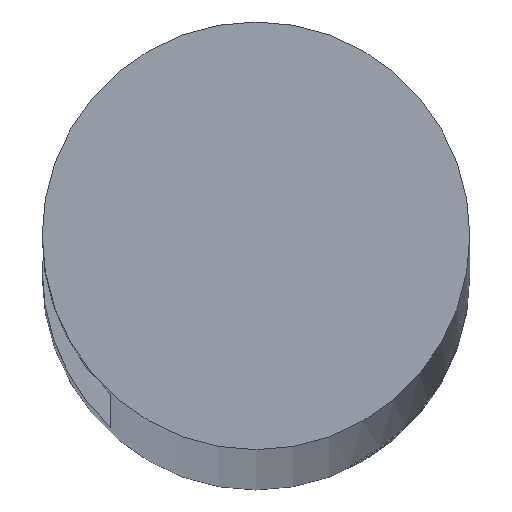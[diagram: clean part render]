
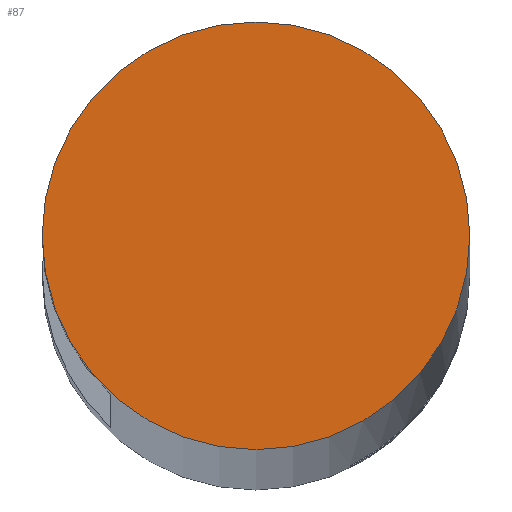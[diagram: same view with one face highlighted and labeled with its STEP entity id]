
A CAD part, top view. The second image highlights one B-rep face of the part: STEP entity #87.
In plain terms, the highlighted planar face has unit normal (0, 0, 1).
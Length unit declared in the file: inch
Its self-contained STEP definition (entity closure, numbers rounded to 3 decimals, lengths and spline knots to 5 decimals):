
#5 = PLANE ( 'NONE',  #377 ) ;
#20 = AXIS2_PLACEMENT_3D ( 'NONE', #104, #286, #144 ) ;
#34 = DIRECTION ( 'NONE',  ( 1., 0., 0. ) ) ;
#66 = CARTESIAN_POINT ( 'NONE',  ( 0., 0., 6.75 ) ) ;
#81 = AXIS2_PLACEMENT_3D ( 'NONE', #359, #93, #325 ) ;
#87 = ADVANCED_FACE ( 'NONE', ( #97 ), #5, .T. ) ;
#93 = DIRECTION ( 'NONE',  ( 0., 0., 1. ) ) ;
#96 = CIRCLE ( 'NONE', #81, 0.0625 ) ;
#97 = FACE_OUTER_BOUND ( 'NONE', #176, .T. ) ;
#104 = CARTESIAN_POINT ( 'NONE',  ( 0., 0., 6.75 ) ) ;
#143 = EDGE_CURVE ( 'NONE', #248, #183, #96, .T. ) ;
#144 = DIRECTION ( 'NONE',  ( 1., 0., 0. ) ) ;
#145 = CIRCLE ( 'NONE', #20, 0.0625 ) ;
#156 = ORIENTED_EDGE ( 'NONE', *, *, #143, .T. ) ;
#176 = EDGE_LOOP ( 'NONE', ( #243, #156 ) ) ;
#183 = VERTEX_POINT ( 'NONE', #242 ) ;
#209 = CARTESIAN_POINT ( 'NONE',  ( 0.0625, 0., 6.75 ) ) ;
#213 = DIRECTION ( 'NONE',  ( 0., 0., 1. ) ) ;
#242 = CARTESIAN_POINT ( 'NONE',  ( -0.0625, 0., 6.75 ) ) ;
#243 = ORIENTED_EDGE ( 'NONE', *, *, #380, .T. ) ;
#248 = VERTEX_POINT ( 'NONE', #209 ) ;
#286 = DIRECTION ( 'NONE',  ( 0., 0., 1. ) ) ;
#325 = DIRECTION ( 'NONE',  ( 1., 0., 0. ) ) ;
#359 = CARTESIAN_POINT ( 'NONE',  ( 0., 0., 6.75 ) ) ;
#377 = AXIS2_PLACEMENT_3D ( 'NONE', #66, #213, #34 ) ;
#380 = EDGE_CURVE ( 'NONE', #183, #248, #145, .T. ) ;
